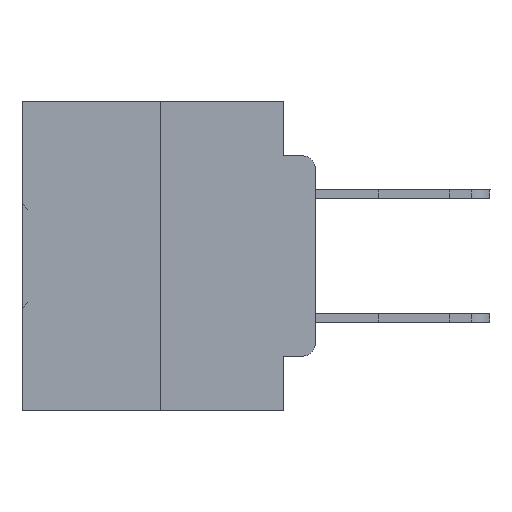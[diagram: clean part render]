
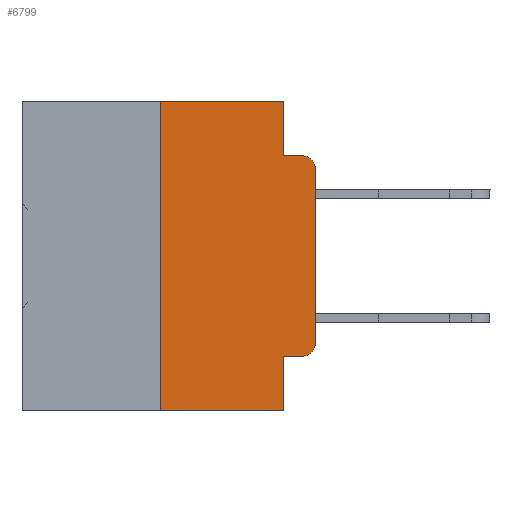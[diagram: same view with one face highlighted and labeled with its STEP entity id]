
A CAD part, left-side view. The second image highlights one B-rep face of the part: STEP entity #6799.
In plain terms, the highlighted planar face has unit normal (-1, 0, 0).
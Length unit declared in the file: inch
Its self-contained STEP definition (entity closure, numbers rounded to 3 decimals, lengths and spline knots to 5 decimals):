
#57 = CARTESIAN_POINT ( 'NONE',  ( 0., 0.25, 0. ) ) ;
#369 = CIRCLE ( 'NONE', #9999, 0.02 ) ;
#1188 = VECTOR ( 'NONE', #24777, 39.37008 ) ;
#1531 = DIRECTION ( 'NONE',  ( 0., 0., -1. ) ) ;
#1688 = ORIENTED_EDGE ( 'NONE', *, *, #20500, .T. ) ;
#2519 = VECTOR ( 'NONE', #13391, 39.37008 ) ;
#3337 = DIRECTION ( 'NONE',  ( 1., 0., 0. ) ) ;
#3762 = LINE ( 'NONE', #28743, #30736 ) ;
#4218 = CARTESIAN_POINT ( 'NONE',  ( 0., 0., -0.1085 ) ) ;
#4347 = CIRCLE ( 'NONE', #17489, 0.02 ) ;
#4654 = DIRECTION ( 'NONE',  ( 0., -1., 0. ) ) ;
#5548 = EDGE_CURVE ( 'NONE', #9425, #17619, #14483, .T. ) ;
#6274 = CARTESIAN_POINT ( 'NONE',  ( 0., 0.473, -0.5 ) ) ;
#6799 = ADVANCED_FACE ( 'NONE', ( #17676 ), #27258, .F. ) ;
#7539 = ORIENTED_EDGE ( 'NONE', *, *, #38312, .F. ) ;
#7547 = ORIENTED_EDGE ( 'NONE', *, *, #30056, .T. ) ;
#8212 = CARTESIAN_POINT ( 'NONE',  ( 0., 0., -0.3915 ) ) ;
#9264 = ORIENTED_EDGE ( 'NONE', *, *, #15168, .F. ) ;
#9425 = VERTEX_POINT ( 'NONE', #24425 ) ;
#9510 = ORIENTED_EDGE ( 'NONE', *, *, #5548, .F. ) ;
#9999 = AXIS2_PLACEMENT_3D ( 'NONE', #25909, #26824, #35022 ) ;
#10375 = LINE ( 'NONE', #28579, #15053 ) ;
#10869 = ORIENTED_EDGE ( 'NONE', *, *, #18365, .T. ) ;
#11578 = ORIENTED_EDGE ( 'NONE', *, *, #38386, .T. ) ;
#12348 = VERTEX_POINT ( 'NONE', #4218 ) ;
#12351 = CARTESIAN_POINT ( 'NONE',  ( 0., 0.25, 0. ) ) ;
#13128 = CARTESIAN_POINT ( 'NONE',  ( 0., 0., 0. ) ) ;
#13301 = DIRECTION ( 'NONE',  ( 0., 0., -1. ) ) ;
#13391 = DIRECTION ( 'NONE',  ( 0., 0., 1. ) ) ;
#13834 = LINE ( 'NONE', #30208, #31483 ) ;
#14174 = DIRECTION ( 'NONE',  ( 0., -1., 0. ) ) ;
#14483 = LINE ( 'NONE', #22158, #17315 ) ;
#15053 = VECTOR ( 'NONE', #4654, 39.37008 ) ;
#15168 = EDGE_CURVE ( 'NONE', #16602, #28868, #3762, .T. ) ;
#15690 = CARTESIAN_POINT ( 'NONE',  ( 0., 0.051, 0. ) ) ;
#16537 = CARTESIAN_POINT ( 'NONE',  ( 0., 0.02, -0.4115 ) ) ;
#16602 = VERTEX_POINT ( 'NONE', #57 ) ;
#16641 = EDGE_CURVE ( 'NONE', #27096, #17619, #18508, .T. ) ;
#17315 = VECTOR ( 'NONE', #13301, 39.37008 ) ;
#17489 = AXIS2_PLACEMENT_3D ( 'NONE', #19359, #34299, #1531 ) ;
#17619 = VERTEX_POINT ( 'NONE', #37448 ) ;
#17676 = FACE_OUTER_BOUND ( 'NONE', #34515, .T. ) ;
#18262 = VERTEX_POINT ( 'NONE', #34399 ) ;
#18365 = EDGE_CURVE ( 'NONE', #35879, #37156, #369, .T. ) ;
#18395 = ORIENTED_EDGE ( 'NONE', *, *, #29687, .F. ) ;
#18508 = LINE ( 'NONE', #6274, #37152 ) ;
#18509 = VERTEX_POINT ( 'NONE', #31344 ) ;
#19276 = DIRECTION ( 'NONE',  ( 0., 0., 1. ) ) ;
#19359 = CARTESIAN_POINT ( 'NONE',  ( 0., 0.02, -0.1085 ) ) ;
#20500 = EDGE_CURVE ( 'NONE', #37156, #12348, #23462, .T. ) ;
#21199 = LINE ( 'NONE', #15690, #1188 ) ;
#21696 = ORIENTED_EDGE ( 'NONE', *, *, #35401, .F. ) ;
#22031 = ORIENTED_EDGE ( 'NONE', *, *, #16641, .T. ) ;
#22158 = CARTESIAN_POINT ( 'NONE',  ( 0., 0.051, 0. ) ) ;
#23462 = LINE ( 'NONE', #13128, #2519 ) ;
#23689 = VECTOR ( 'NONE', #19276, 39.37008 ) ;
#24425 = CARTESIAN_POINT ( 'NONE',  ( 0., 0.051, -0.4115 ) ) ;
#24777 = DIRECTION ( 'NONE',  ( 0., 0., -1. ) ) ;
#25909 = CARTESIAN_POINT ( 'NONE',  ( 0., 0.02, -0.3915 ) ) ;
#26351 = CARTESIAN_POINT ( 'NONE',  ( 0., 0.051, 0. ) ) ;
#26824 = DIRECTION ( 'NONE',  ( -1., 0., 0. ) ) ;
#27096 = VERTEX_POINT ( 'NONE', #37925 ) ;
#27258 = PLANE ( 'NONE',  #36046 ) ;
#28579 = CARTESIAN_POINT ( 'NONE',  ( 0., 0.051, -0.0885 ) ) ;
#28743 = CARTESIAN_POINT ( 'NONE',  ( 0., 0.473, 0. ) ) ;
#28868 = VERTEX_POINT ( 'NONE', #26351 ) ;
#29687 = EDGE_CURVE ( 'NONE', #28868, #18262, #21199, .T. ) ;
#29832 = DIRECTION ( 'NONE',  ( 0., -1., 0. ) ) ;
#30056 = EDGE_CURVE ( 'NONE', #9425, #35879, #13834, .T. ) ;
#30208 = CARTESIAN_POINT ( 'NONE',  ( 0., 0.051, -0.4115 ) ) ;
#30736 = VECTOR ( 'NONE', #14174, 39.37008 ) ;
#31344 = CARTESIAN_POINT ( 'NONE',  ( 0., 0.02, -0.0885 ) ) ;
#31483 = VECTOR ( 'NONE', #38045, 39.37008 ) ;
#32504 = LINE ( 'NONE', #12351, #23689 ) ;
#34299 = DIRECTION ( 'NONE',  ( -1., 0., 0. ) ) ;
#34399 = CARTESIAN_POINT ( 'NONE',  ( 0., 0.051, -0.0885 ) ) ;
#34515 = EDGE_LOOP ( 'NONE', ( #1688, #11578, #7539, #18395, #9264, #21696, #22031, #9510, #7547, #10869 ) ) ;
#35022 = DIRECTION ( 'NONE',  ( 0., 0., -1. ) ) ;
#35401 = EDGE_CURVE ( 'NONE', #27096, #16602, #32504, .T. ) ;
#35879 = VERTEX_POINT ( 'NONE', #16537 ) ;
#36046 = AXIS2_PLACEMENT_3D ( 'NONE', #36512, #3337, #36122 ) ;
#36122 = DIRECTION ( 'NONE',  ( 0., 0., -1. ) ) ;
#36512 = CARTESIAN_POINT ( 'NONE',  ( 0., 0.473, 0. ) ) ;
#37152 = VECTOR ( 'NONE', #29832, 39.37008 ) ;
#37156 = VERTEX_POINT ( 'NONE', #8212 ) ;
#37448 = CARTESIAN_POINT ( 'NONE',  ( 0., 0.051, -0.5 ) ) ;
#37925 = CARTESIAN_POINT ( 'NONE',  ( 0., 0.25, -0.5 ) ) ;
#38045 = DIRECTION ( 'NONE',  ( 0., -1., 0. ) ) ;
#38312 = EDGE_CURVE ( 'NONE', #18262, #18509, #10375, .T. ) ;
#38386 = EDGE_CURVE ( 'NONE', #12348, #18509, #4347, .T. ) ;
